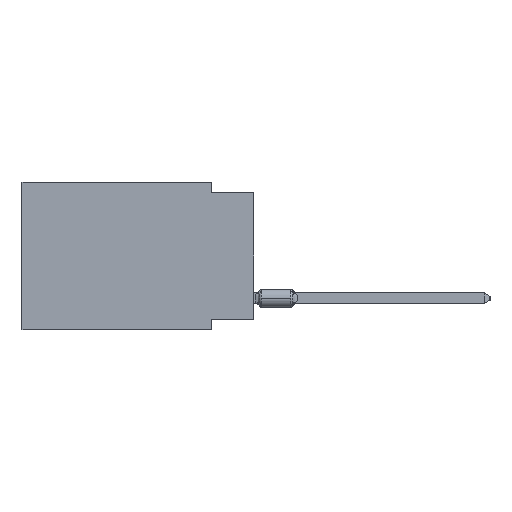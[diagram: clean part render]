
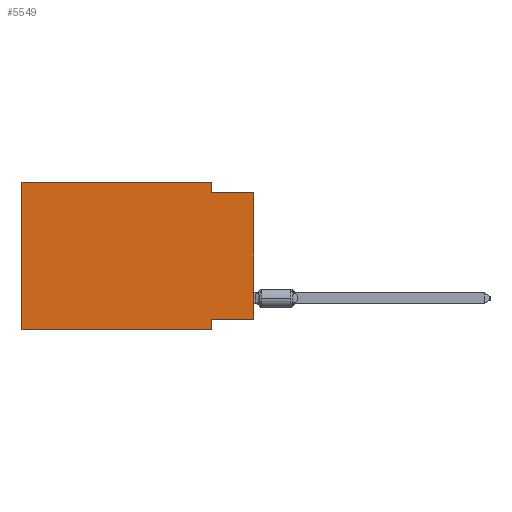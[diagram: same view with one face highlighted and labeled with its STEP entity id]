
A CAD part, left-side view. The second image highlights one B-rep face of the part: STEP entity #5549.
In plain terms, the highlighted planar face has unit normal (-1, 0, 0).
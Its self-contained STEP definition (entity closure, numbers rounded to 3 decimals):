
#1505 = VERTEX_POINT ( 'NONE', #1720 ) ;
#1540 = ORIENTED_EDGE ( 'NONE', *, *, #73526, .F. ) ;
#1549 = VERTEX_POINT ( 'NONE', #72953 ) ;
#1720 = CARTESIAN_POINT ( 'NONE',  ( 0., 2.54, -8.89 ) ) ;
#3269 = CARTESIAN_POINT ( 'NONE',  ( 0., 13.97, -8.89 ) ) ;
#4706 = LINE ( 'NONE', #17653, #30953 ) ;
#4713 = VECTOR ( 'NONE', #35805, 1000. ) ;
#5549 = ADVANCED_FACE ( 'NONE', ( #65074 ), #12492, .F. ) ;
#5703 = CARTESIAN_POINT ( 'NONE',  ( 0., 2.54, 0. ) ) ;
#5973 = DIRECTION ( 'NONE',  ( 0., 0., 1. ) ) ;
#6371 = DIRECTION ( 'NONE',  ( 0., -1., 0. ) ) ;
#7470 = CARTESIAN_POINT ( 'NONE',  ( 0., 0., -8.255 ) ) ;
#10329 = EDGE_CURVE ( 'NONE', #17705, #1505, #16038, .T. ) ;
#11209 = LINE ( 'NONE', #11954, #68919 ) ;
#11954 = CARTESIAN_POINT ( 'NONE',  ( 0., 2.54, -8.89 ) ) ;
#12108 = DIRECTION ( 'NONE',  ( 1., 0., 0. ) ) ;
#12492 = PLANE ( 'NONE',  #38904 ) ;
#13016 = CARTESIAN_POINT ( 'NONE',  ( 0., 2.54, -0.635 ) ) ;
#16038 = LINE ( 'NONE', #22876, #61138 ) ;
#17653 = CARTESIAN_POINT ( 'NONE',  ( 0., 0., -8.255 ) ) ;
#17705 = VERTEX_POINT ( 'NONE', #3269 ) ;
#18358 = LINE ( 'NONE', #41601, #33759 ) ;
#18584 = LINE ( 'NONE', #70413, #29335 ) ;
#21008 = EDGE_CURVE ( 'NONE', #17705, #1549, #18358, .T. ) ;
#22876 = CARTESIAN_POINT ( 'NONE',  ( 0., 13.97, -8.89 ) ) ;
#23124 = CARTESIAN_POINT ( 'NONE',  ( 0., 0., 0. ) ) ;
#28839 = LINE ( 'NONE', #23124, #54136 ) ;
#29260 = DIRECTION ( 'NONE',  ( 0., -1., 0. ) ) ;
#29335 = VECTOR ( 'NONE', #29260, 1000. ) ;
#30603 = VERTEX_POINT ( 'NONE', #7470 ) ;
#30953 = VECTOR ( 'NONE', #75202, 1000. ) ;
#31849 = CARTESIAN_POINT ( 'NONE',  ( 0., 2.54, -8.255 ) ) ;
#32261 = EDGE_LOOP ( 'NONE', ( #69800, #35230, #52994, #72231, #58797, #71113, #62497, #1540 ) ) ;
#33759 = VECTOR ( 'NONE', #59120, 1000. ) ;
#35200 = DIRECTION ( 'NONE',  ( 0., 0., -1. ) ) ;
#35230 = ORIENTED_EDGE ( 'NONE', *, *, #51553, .F. ) ;
#35331 = LINE ( 'NONE', #58563, #36605 ) ;
#35805 = DIRECTION ( 'NONE',  ( 0., 0., -1. ) ) ;
#36177 = EDGE_CURVE ( 'NONE', #69631, #1505, #11209, .T. ) ;
#36605 = VECTOR ( 'NONE', #6371, 1000. ) ;
#38904 = AXIS2_PLACEMENT_3D ( 'NONE', #53995, #12108, #59719 ) ;
#41601 = CARTESIAN_POINT ( 'NONE',  ( 0., 13.97, 0. ) ) ;
#42125 = CARTESIAN_POINT ( 'NONE',  ( 0., 0., -0.635 ) ) ;
#51553 = EDGE_CURVE ( 'NONE', #69125, #59094, #18584, .T. ) ;
#52994 = ORIENTED_EDGE ( 'NONE', *, *, #66760, .F. ) ;
#53995 = CARTESIAN_POINT ( 'NONE',  ( 0., 13.97, 0. ) ) ;
#54136 = VECTOR ( 'NONE', #5973, 1000. ) ;
#55223 = VERTEX_POINT ( 'NONE', #59327 ) ;
#56720 = EDGE_CURVE ( 'NONE', #30603, #59094, #28839, .T. ) ;
#58563 = CARTESIAN_POINT ( 'NONE',  ( 0., 13.97, 0. ) ) ;
#58797 = ORIENTED_EDGE ( 'NONE', *, *, #21008, .F. ) ;
#59094 = VERTEX_POINT ( 'NONE', #42125 ) ;
#59120 = DIRECTION ( 'NONE',  ( 0., 0., 1. ) ) ;
#59327 = CARTESIAN_POINT ( 'NONE',  ( 0., 2.54, 0. ) ) ;
#59719 = DIRECTION ( 'NONE',  ( 0., 0., -1. ) ) ;
#61138 = VECTOR ( 'NONE', #73586, 1000. ) ;
#62497 = ORIENTED_EDGE ( 'NONE', *, *, #36177, .F. ) ;
#65074 = FACE_OUTER_BOUND ( 'NONE', #32261, .T. ) ;
#66760 = EDGE_CURVE ( 'NONE', #55223, #69125, #69741, .T. ) ;
#68919 = VECTOR ( 'NONE', #35200, 1000. ) ;
#69125 = VERTEX_POINT ( 'NONE', #13016 ) ;
#69429 = EDGE_CURVE ( 'NONE', #1549, #55223, #35331, .T. ) ;
#69631 = VERTEX_POINT ( 'NONE', #31849 ) ;
#69741 = LINE ( 'NONE', #5703, #4713 ) ;
#69800 = ORIENTED_EDGE ( 'NONE', *, *, #56720, .T. ) ;
#70413 = CARTESIAN_POINT ( 'NONE',  ( 0., 0., -0.635 ) ) ;
#71113 = ORIENTED_EDGE ( 'NONE', *, *, #10329, .T. ) ;
#72231 = ORIENTED_EDGE ( 'NONE', *, *, #69429, .F. ) ;
#72953 = CARTESIAN_POINT ( 'NONE',  ( 0., 13.97, 0. ) ) ;
#73526 = EDGE_CURVE ( 'NONE', #30603, #69631, #4706, .T. ) ;
#73586 = DIRECTION ( 'NONE',  ( 0., -1., 0. ) ) ;
#75202 = DIRECTION ( 'NONE',  ( 0., 1., 0. ) ) ;
